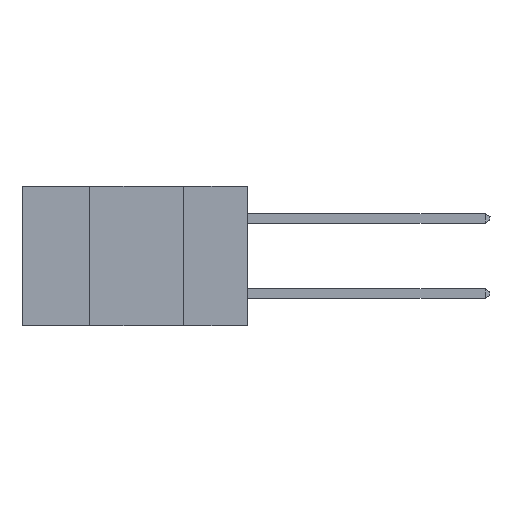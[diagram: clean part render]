
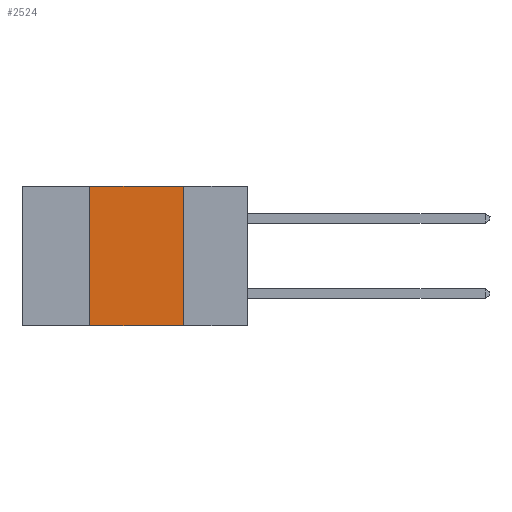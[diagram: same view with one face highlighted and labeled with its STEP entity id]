
A CAD part, left-side view. The second image highlights one B-rep face of the part: STEP entity #2524.
In plain terms, the highlighted planar face has unit normal (-1, 0, 0).
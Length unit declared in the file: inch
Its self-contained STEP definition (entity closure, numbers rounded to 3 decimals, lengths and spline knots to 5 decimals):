
#1462 = DIRECTION ( 'NONE',  ( 0., 0., 1. ) ) ;
#2304 = EDGE_CURVE ( 'NONE', #5578, #8449, #3114, .T. ) ;
#2451 = CARTESIAN_POINT ( 'NONE',  ( 0., 0.17, 0. ) ) ;
#2524 = ADVANCED_FACE ( 'NONE', ( #17511 ), #11666, .F. ) ;
#2554 = AXIS2_PLACEMENT_3D ( 'NONE', #17239, #4778, #3301 ) ;
#2672 = VECTOR ( 'NONE', #3412, 39.37008 ) ;
#3114 = LINE ( 'NONE', #10023, #3135 ) ;
#3135 = VECTOR ( 'NONE', #1462, 39.37008 ) ;
#3301 = DIRECTION ( 'NONE',  ( 0., 0., -1. ) ) ;
#3412 = DIRECTION ( 'NONE',  ( 0., -1., 0. ) ) ;
#3695 = LINE ( 'NONE', #15050, #11868 ) ;
#3888 = DIRECTION ( 'NONE',  ( 0., 0., -1. ) ) ;
#3964 = DIRECTION ( 'NONE',  ( 0., -1., 0. ) ) ;
#4597 = EDGE_CURVE ( 'NONE', #11595, #10842, #17289, .T. ) ;
#4778 = DIRECTION ( 'NONE',  ( 1., 0., 0. ) ) ;
#4795 = LINE ( 'NONE', #10403, #2672 ) ;
#5578 = VERTEX_POINT ( 'NONE', #11471 ) ;
#6366 = CARTESIAN_POINT ( 'NONE',  ( 0., 0.42, 0. ) ) ;
#6635 = EDGE_CURVE ( 'NONE', #5578, #10842, #4795, .T. ) ;
#7424 = ORIENTED_EDGE ( 'NONE', *, *, #2304, .F. ) ;
#8449 = VERTEX_POINT ( 'NONE', #6366 ) ;
#8607 = ORIENTED_EDGE ( 'NONE', *, *, #15247, .F. ) ;
#9691 = CARTESIAN_POINT ( 'NONE',  ( 0., 0.17, -0.37 ) ) ;
#9718 = EDGE_LOOP ( 'NONE', ( #15906, #8607, #7424, #17172 ) ) ;
#9956 = VECTOR ( 'NONE', #3888, 39.37008 ) ;
#10023 = CARTESIAN_POINT ( 'NONE',  ( 0., 0.42, -0.37 ) ) ;
#10403 = CARTESIAN_POINT ( 'NONE',  ( 0., 0.6, -0.37 ) ) ;
#10842 = VERTEX_POINT ( 'NONE', #9691 ) ;
#11471 = CARTESIAN_POINT ( 'NONE',  ( 0., 0.42, -0.37 ) ) ;
#11595 = VERTEX_POINT ( 'NONE', #2451 ) ;
#11666 = PLANE ( 'NONE',  #2554 ) ;
#11868 = VECTOR ( 'NONE', #3964, 39.37008 ) ;
#14538 = CARTESIAN_POINT ( 'NONE',  ( 0., 0.17, -0.37 ) ) ;
#15050 = CARTESIAN_POINT ( 'NONE',  ( 0., 0.6, 0. ) ) ;
#15247 = EDGE_CURVE ( 'NONE', #8449, #11595, #3695, .T. ) ;
#15906 = ORIENTED_EDGE ( 'NONE', *, *, #4597, .F. ) ;
#17172 = ORIENTED_EDGE ( 'NONE', *, *, #6635, .T. ) ;
#17239 = CARTESIAN_POINT ( 'NONE',  ( 0., 0.6, 0. ) ) ;
#17289 = LINE ( 'NONE', #14538, #9956 ) ;
#17511 = FACE_OUTER_BOUND ( 'NONE', #9718, .T. ) ;
